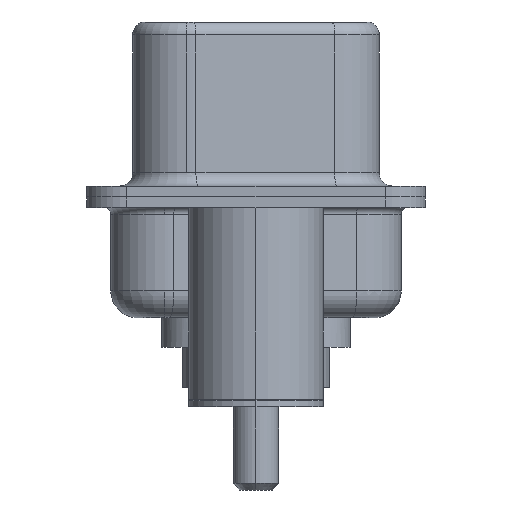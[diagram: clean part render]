
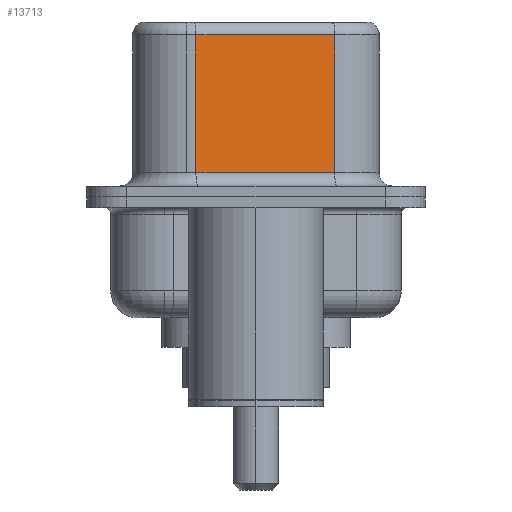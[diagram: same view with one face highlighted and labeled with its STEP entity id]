
A CAD part, left-side view. The second image highlights one B-rep face of the part: STEP entity #13713.
In plain terms, the highlighted planar face has unit normal (-0.985, -0.174, 0).
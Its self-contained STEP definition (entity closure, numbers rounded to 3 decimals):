
#951 = LINE ( 'NONE', #2449, #12305 ) ;
#1235 = DIRECTION ( 'NONE',  ( 0., 0., -1. ) ) ;
#1611 = EDGE_CURVE ( 'NONE', #8112, #13440, #5615, .T. ) ;
#2199 = EDGE_LOOP ( 'NONE', ( #8467, #3273, #15236, #3053 ) ) ;
#2449 = CARTESIAN_POINT ( 'NONE',  ( 4.585, -2.927, 0.9 ) ) ;
#2944 = VERTEX_POINT ( 'NONE', #10221 ) ;
#3053 = ORIENTED_EDGE ( 'NONE', *, *, #13132, .T. ) ;
#3273 = ORIENTED_EDGE ( 'NONE', *, *, #5983, .T. ) ;
#4235 = CARTESIAN_POINT ( 'NONE',  ( 3.675, 2.233, 6.52 ) ) ;
#4304 = CARTESIAN_POINT ( 'NONE',  ( 3.675, 2.233, 6.02 ) ) ;
#4400 = PLANE ( 'NONE',  #5340 ) ;
#4418 = VECTOR ( 'NONE', #1235, 1000. ) ;
#4821 = VERTEX_POINT ( 'NONE', #7490 ) ;
#5340 = AXIS2_PLACEMENT_3D ( 'NONE', #14448, #15768, #7336 ) ;
#5615 = LINE ( 'NONE', #4235, #6067 ) ;
#5983 = EDGE_CURVE ( 'NONE', #4821, #8112, #7966, .T. ) ;
#6067 = VECTOR ( 'NONE', #8878, 1000. ) ;
#7336 = DIRECTION ( 'NONE',  ( -0.174, 0.985, 0. ) ) ;
#7490 = CARTESIAN_POINT ( 'NONE',  ( 4.585, -2.927, 6.02 ) ) ;
#7966 = LINE ( 'NONE', #14263, #18130 ) ;
#8112 = VERTEX_POINT ( 'NONE', #4304 ) ;
#8292 = LINE ( 'NONE', #11623, #4418 ) ;
#8467 = ORIENTED_EDGE ( 'NONE', *, *, #12252, .F. ) ;
#8878 = DIRECTION ( 'NONE',  ( 0., 0., -1. ) ) ;
#10221 = CARTESIAN_POINT ( 'NONE',  ( 4.585, -2.927, 0.9 ) ) ;
#11200 = DIRECTION ( 'NONE',  ( 0.174, -0.985, 0. ) ) ;
#11623 = CARTESIAN_POINT ( 'NONE',  ( 4.585, -2.927, 6.52 ) ) ;
#11654 = CARTESIAN_POINT ( 'NONE',  ( 3.675, 2.233, 0.9 ) ) ;
#12252 = EDGE_CURVE ( 'NONE', #4821, #2944, #8292, .T. ) ;
#12305 = VECTOR ( 'NONE', #11200, 1000. ) ;
#13132 = EDGE_CURVE ( 'NONE', #13440, #2944, #951, .T. ) ;
#13440 = VERTEX_POINT ( 'NONE', #11654 ) ;
#13713 = ADVANCED_FACE ( 'NONE', ( #16343 ), #4400, .F. ) ;
#14263 = CARTESIAN_POINT ( 'NONE',  ( 4.585, -2.927, 6.02 ) ) ;
#14448 = CARTESIAN_POINT ( 'NONE',  ( 4.585, -2.927, 6.52 ) ) ;
#15236 = ORIENTED_EDGE ( 'NONE', *, *, #1611, .T. ) ;
#15768 = DIRECTION ( 'NONE',  ( 0.985, 0.174, 0. ) ) ;
#16343 = FACE_OUTER_BOUND ( 'NONE', #2199, .T. ) ;
#17630 = DIRECTION ( 'NONE',  ( -0.174, 0.985, 0. ) ) ;
#18130 = VECTOR ( 'NONE', #17630, 1000. ) ;
